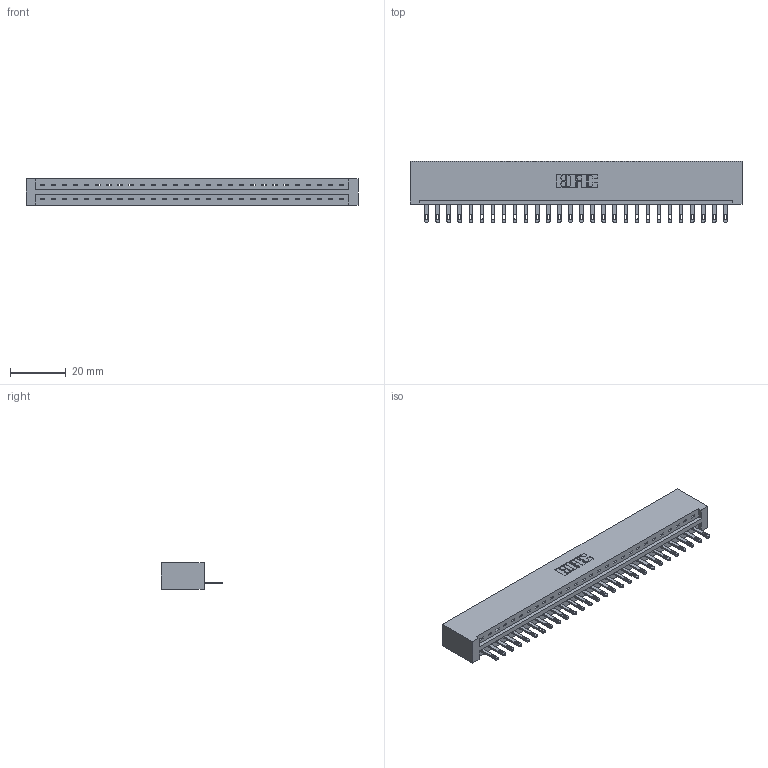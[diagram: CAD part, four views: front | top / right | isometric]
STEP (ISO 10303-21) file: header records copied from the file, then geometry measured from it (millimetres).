
FILE_DESCRIPTION (( 'STEP AP203' ), '1' );
FILE_NAME ('337-028-500-101.STEP', '2019-09-30T20:22:25', ( '' ), ( '' ), 'SwSTEP 2.0', 'SolidWorks 2016', '' );
FILE_SCHEMA (( 'CONFIG_CONTROL_DESIGN' ));
Length unit declared in the file: inch
Products named in the file (3): 337-028-500-101; 337 Part_No Mounting Lugs; 345-292-001_345-293-100
Assembly tree (29 placements, depth 2):
  337-028-500-101
    337 Part_No Mounting Lugs
    345-292-001_345-293-100  x28
Bounding box: 118.82 x 21.85 x 9.4 mm (x, y, z)
Volume: 12930.3 mm3; surface area: 13330.7 mm2
Topology: 29 solids, 29 shells, 1730 faces, 5327 edges, 3550 vertices
Faces by surface type: plane 1186, cylinder 544
Entity records: 22277 total; most frequent: CARTESIAN_POINT 3886, ORIENTED_EDGE 3850, DIRECTION 3293, EDGE_CURVE 1925, VECTOR 1801, LINE 1801, VERTEX_POINT 1282, AXIS2_PLACEMENT_3D 746
